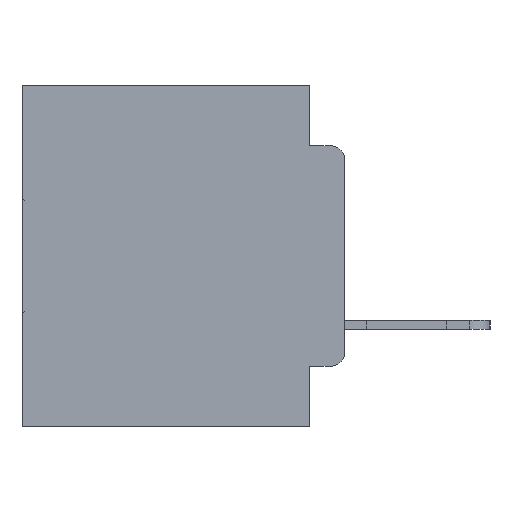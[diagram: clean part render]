
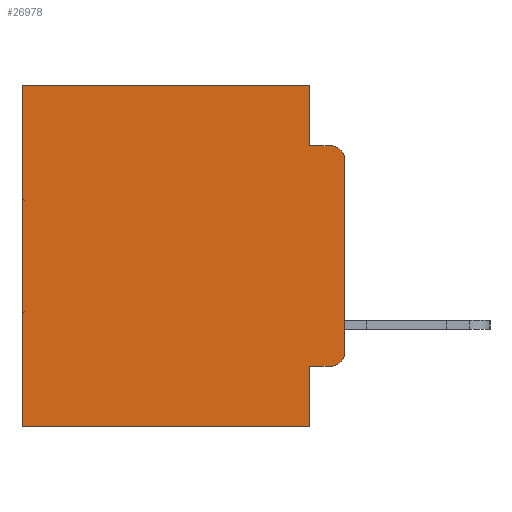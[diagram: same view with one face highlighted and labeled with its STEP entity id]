
A CAD part, left-side view. The second image highlights one B-rep face of the part: STEP entity #26978.
In plain terms, the highlighted planar face has unit normal (-1, 0, 0).
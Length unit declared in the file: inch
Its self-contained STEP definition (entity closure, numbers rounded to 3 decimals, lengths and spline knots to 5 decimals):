
#75 = DIRECTION ( 'NONE',  ( 0., 1., 0. ) ) ;
#157 = DIRECTION ( 'NONE',  ( 0., 0., -1. ) ) ;
#439 = CARTESIAN_POINT ( 'NONE',  ( 0.298, 0.051, 0. ) ) ;
#812 = ORIENTED_EDGE ( 'NONE', *, *, #15420, .T. ) ;
#1506 = DIRECTION ( 'NONE',  ( 0., -1., 0. ) ) ;
#2881 = CARTESIAN_POINT ( 'NONE',  ( 0.298, 0.051, 0. ) ) ;
#3025 = PLANE ( 'NONE',  #13633 ) ;
#3104 = CARTESIAN_POINT ( 'NONE',  ( 0.298, 0.02, -0.0885 ) ) ;
#3469 = AXIS2_PLACEMENT_3D ( 'NONE', #17148, #17847, #17826 ) ;
#3635 = LINE ( 'NONE', #10351, #29001 ) ;
#3887 = EDGE_CURVE ( 'NONE', #9096, #6019, #10143, .T. ) ;
#4230 = ORIENTED_EDGE ( 'NONE', *, *, #7315, .F. ) ;
#4844 = VERTEX_POINT ( 'NONE', #16485 ) ;
#5000 = ORIENTED_EDGE ( 'NONE', *, *, #15021, .T. ) ;
#5613 = DIRECTION ( 'NONE',  ( 1., 0., 0. ) ) ;
#6019 = VERTEX_POINT ( 'NONE', #3104 ) ;
#6252 = EDGE_CURVE ( 'NONE', #18262, #31846, #13534, .T. ) ;
#6503 = CARTESIAN_POINT ( 'NONE',  ( 0.298, 0.02, -0.3915 ) ) ;
#6571 = DIRECTION ( 'NONE',  ( 0., 0., -1. ) ) ;
#6830 = LINE ( 'NONE', #22711, #18604 ) ;
#7090 = VECTOR ( 'NONE', #18553, 39.37008 ) ;
#7315 = EDGE_CURVE ( 'NONE', #9096, #25271, #21940, .T. ) ;
#7398 = ORIENTED_EDGE ( 'NONE', *, *, #13658, .F. ) ;
#7911 = VERTEX_POINT ( 'NONE', #28755 ) ;
#8372 = CARTESIAN_POINT ( 'NONE',  ( 0.298, 0., -0.5 ) ) ;
#8892 = LINE ( 'NONE', #2881, #14855 ) ;
#9096 = VERTEX_POINT ( 'NONE', #15545 ) ;
#9156 = ORIENTED_EDGE ( 'NONE', *, *, #21137, .F. ) ;
#9607 = CIRCLE ( 'NONE', #12575, 0.02 ) ;
#9791 = ORIENTED_EDGE ( 'NONE', *, *, #17903, .F. ) ;
#10143 = CIRCLE ( 'NONE', #3469, 0.02 ) ;
#10263 = VECTOR ( 'NONE', #25177, 39.37008 ) ;
#10351 = CARTESIAN_POINT ( 'NONE',  ( 0.298, 0., 0. ) ) ;
#11051 = LINE ( 'NONE', #15721, #10263 ) ;
#11538 = CARTESIAN_POINT ( 'NONE',  ( 0.298, 0.473, 0. ) ) ;
#11942 = ORIENTED_EDGE ( 'NONE', *, *, #3887, .T. ) ;
#12160 = CARTESIAN_POINT ( 'NONE',  ( 0.298, 0., 0. ) ) ;
#12575 = AXIS2_PLACEMENT_3D ( 'NONE', #6503, #31643, #6571 ) ;
#13534 = LINE ( 'NONE', #20296, #24900 ) ;
#13633 = AXIS2_PLACEMENT_3D ( 'NONE', #18166, #5613, #22985 ) ;
#13658 = EDGE_CURVE ( 'NONE', #15449, #7911, #20267, .T. ) ;
#14834 = VERTEX_POINT ( 'NONE', #11538 ) ;
#14855 = VECTOR ( 'NONE', #27139, 39.37008 ) ;
#15021 = EDGE_CURVE ( 'NONE', #31846, #25271, #9607, .T. ) ;
#15420 = EDGE_CURVE ( 'NONE', #14834, #4844, #6830, .T. ) ;
#15449 = VERTEX_POINT ( 'NONE', #20309 ) ;
#15545 = CARTESIAN_POINT ( 'NONE',  ( 0.298, 0., -0.1085 ) ) ;
#15721 = CARTESIAN_POINT ( 'NONE',  ( 0.298, 0.051, -0.0885 ) ) ;
#16000 = CARTESIAN_POINT ( 'NONE',  ( 0.298, 0.051, -0.4115 ) ) ;
#16485 = CARTESIAN_POINT ( 'NONE',  ( 0.298, 0.473, -0.5 ) ) ;
#16639 = ORIENTED_EDGE ( 'NONE', *, *, #18757, .T. ) ;
#17118 = ORIENTED_EDGE ( 'NONE', *, *, #23254, .F. ) ;
#17148 = CARTESIAN_POINT ( 'NONE',  ( 0.298, 0.02, -0.1085 ) ) ;
#17514 = DIRECTION ( 'NONE',  ( 0., 0., -1. ) ) ;
#17826 = DIRECTION ( 'NONE',  ( 0., 0., -1. ) ) ;
#17847 = DIRECTION ( 'NONE',  ( -1., 0., 0. ) ) ;
#17903 = EDGE_CURVE ( 'NONE', #18262, #22270, #8892, .T. ) ;
#18166 = CARTESIAN_POINT ( 'NONE',  ( 0.298, 0., 0. ) ) ;
#18262 = VERTEX_POINT ( 'NONE', #16000 ) ;
#18553 = DIRECTION ( 'NONE',  ( 0., 1., 0. ) ) ;
#18604 = VECTOR ( 'NONE', #22508, 39.37008 ) ;
#18757 = EDGE_CURVE ( 'NONE', #15449, #14834, #3635, .T. ) ;
#20267 = LINE ( 'NONE', #439, #31277 ) ;
#20296 = CARTESIAN_POINT ( 'NONE',  ( 0.298, 0.051, -0.4115 ) ) ;
#20309 = CARTESIAN_POINT ( 'NONE',  ( 0.298, 0.051, 0. ) ) ;
#21137 = EDGE_CURVE ( 'NONE', #7911, #6019, #11051, .T. ) ;
#21940 = LINE ( 'NONE', #12160, #27441 ) ;
#22270 = VERTEX_POINT ( 'NONE', #24513 ) ;
#22508 = DIRECTION ( 'NONE',  ( 0., 0., -1. ) ) ;
#22711 = CARTESIAN_POINT ( 'NONE',  ( 0.298, 0.473, 0. ) ) ;
#22753 = CARTESIAN_POINT ( 'NONE',  ( 0.298, 0.02, -0.4115 ) ) ;
#22985 = DIRECTION ( 'NONE',  ( 0., 0., -1. ) ) ;
#23254 = EDGE_CURVE ( 'NONE', #22270, #4844, #25876, .T. ) ;
#24513 = CARTESIAN_POINT ( 'NONE',  ( 0.298, 0.051, -0.5 ) ) ;
#24900 = VECTOR ( 'NONE', #1506, 39.37008 ) ;
#25177 = DIRECTION ( 'NONE',  ( 0., -1., 0. ) ) ;
#25271 = VERTEX_POINT ( 'NONE', #26835 ) ;
#25876 = LINE ( 'NONE', #8372, #7090 ) ;
#26835 = CARTESIAN_POINT ( 'NONE',  ( 0.298, 0., -0.3915 ) ) ;
#26978 = ADVANCED_FACE ( 'NONE', ( #28602 ), #3025, .F. ) ;
#27139 = DIRECTION ( 'NONE',  ( 0., 0., -1. ) ) ;
#27441 = VECTOR ( 'NONE', #17514, 39.37008 ) ;
#28602 = FACE_OUTER_BOUND ( 'NONE', #31714, .T. ) ;
#28755 = CARTESIAN_POINT ( 'NONE',  ( 0.298, 0.051, -0.0885 ) ) ;
#29001 = VECTOR ( 'NONE', #75, 39.37008 ) ;
#31277 = VECTOR ( 'NONE', #157, 39.37008 ) ;
#31643 = DIRECTION ( 'NONE',  ( -1., 0., 0. ) ) ;
#31685 = ORIENTED_EDGE ( 'NONE', *, *, #6252, .T. ) ;
#31714 = EDGE_LOOP ( 'NONE', ( #4230, #11942, #9156, #7398, #16639, #812, #17118, #9791, #31685, #5000 ) ) ;
#31846 = VERTEX_POINT ( 'NONE', #22753 ) ;
